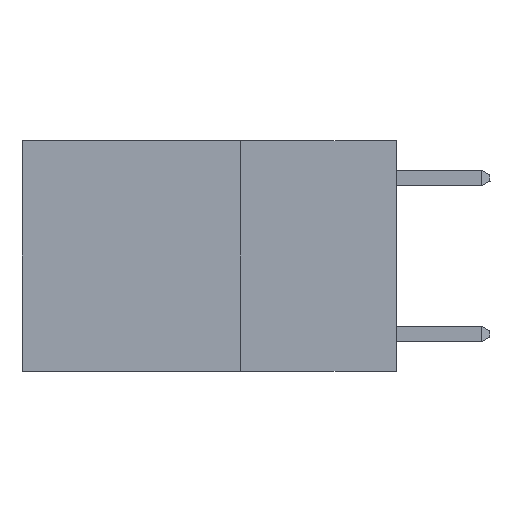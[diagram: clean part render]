
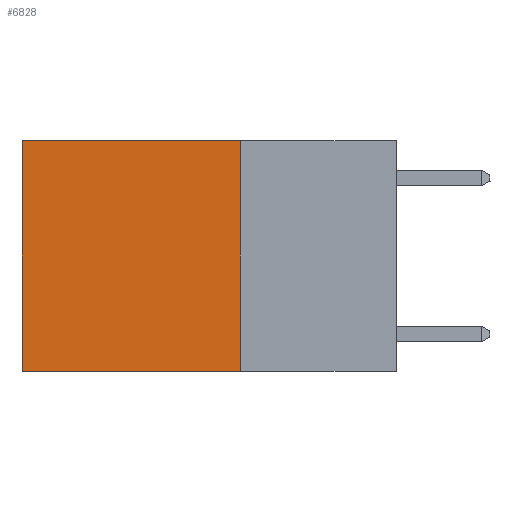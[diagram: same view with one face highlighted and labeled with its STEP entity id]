
A CAD part, left-side view. The second image highlights one B-rep face of the part: STEP entity #6828.
In plain terms, the highlighted planar face has unit normal (-1, 0, 0).
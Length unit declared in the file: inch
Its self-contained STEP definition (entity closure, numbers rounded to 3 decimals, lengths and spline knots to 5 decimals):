
#317 = DIRECTION ( 'NONE',  ( 1., 0., 0. ) ) ;
#559 = FACE_OUTER_BOUND ( 'NONE', #3598, .T. ) ;
#1154 = CARTESIAN_POINT ( 'NONE',  ( 0.2625, 0.25, 0. ) ) ;
#1364 = PLANE ( 'NONE',  #7914 ) ;
#1539 = DIRECTION ( 'NONE',  ( 0., 1., 0. ) ) ;
#1543 = DIRECTION ( 'NONE',  ( 0., 1., 0. ) ) ;
#1567 = ORIENTED_EDGE ( 'NONE', *, *, #5586, .F. ) ;
#1794 = VECTOR ( 'NONE', #1543, 39.37008 ) ;
#1837 = CARTESIAN_POINT ( 'NONE',  ( 0.2625, 0.6, 0. ) ) ;
#1870 = VERTEX_POINT ( 'NONE', #6152 ) ;
#1929 = EDGE_CURVE ( 'NONE', #7314, #9312, #4540, .T. ) ;
#2204 = CARTESIAN_POINT ( 'NONE',  ( 0.2625, 0.25, 0. ) ) ;
#2708 = VECTOR ( 'NONE', #5512, 39.37008 ) ;
#3446 = VECTOR ( 'NONE', #6923, 39.37008 ) ;
#3581 = LINE ( 'NONE', #8417, #7622 ) ;
#3598 = EDGE_LOOP ( 'NONE', ( #6676, #7245, #1567, #8874 ) ) ;
#4540 = LINE ( 'NONE', #8446, #1794 ) ;
#4658 = CARTESIAN_POINT ( 'NONE',  ( 0.2625, 0.6, 0. ) ) ;
#4705 = LINE ( 'NONE', #8619, #2708 ) ;
#5341 = VERTEX_POINT ( 'NONE', #8183 ) ;
#5512 = DIRECTION ( 'NONE',  ( 0., 0., -1. ) ) ;
#5586 = EDGE_CURVE ( 'NONE', #7314, #1870, #4705, .T. ) ;
#6152 = CARTESIAN_POINT ( 'NONE',  ( 0.2625, 0.25, -0.37 ) ) ;
#6676 = ORIENTED_EDGE ( 'NONE', *, *, #7848, .T. ) ;
#6828 = ADVANCED_FACE ( 'NONE', ( #559 ), #1364, .F. ) ;
#6923 = DIRECTION ( 'NONE',  ( 0., 0., -1. ) ) ;
#7245 = ORIENTED_EDGE ( 'NONE', *, *, #8682, .F. ) ;
#7314 = VERTEX_POINT ( 'NONE', #2204 ) ;
#7622 = VECTOR ( 'NONE', #1539, 39.37008 ) ;
#7848 = EDGE_CURVE ( 'NONE', #9312, #5341, #8117, .T. ) ;
#7914 = AXIS2_PLACEMENT_3D ( 'NONE', #1154, #317, #8011 ) ;
#8011 = DIRECTION ( 'NONE',  ( 0., 0., -1. ) ) ;
#8117 = LINE ( 'NONE', #4658, #3446 ) ;
#8183 = CARTESIAN_POINT ( 'NONE',  ( 0.2625, 0.6, -0.37 ) ) ;
#8417 = CARTESIAN_POINT ( 'NONE',  ( 0.2625, 0.25, -0.37 ) ) ;
#8446 = CARTESIAN_POINT ( 'NONE',  ( 0.2625, 0.25, 0. ) ) ;
#8619 = CARTESIAN_POINT ( 'NONE',  ( 0.2625, 0.25, 0. ) ) ;
#8682 = EDGE_CURVE ( 'NONE', #1870, #5341, #3581, .T. ) ;
#8874 = ORIENTED_EDGE ( 'NONE', *, *, #1929, .T. ) ;
#9312 = VERTEX_POINT ( 'NONE', #1837 ) ;
